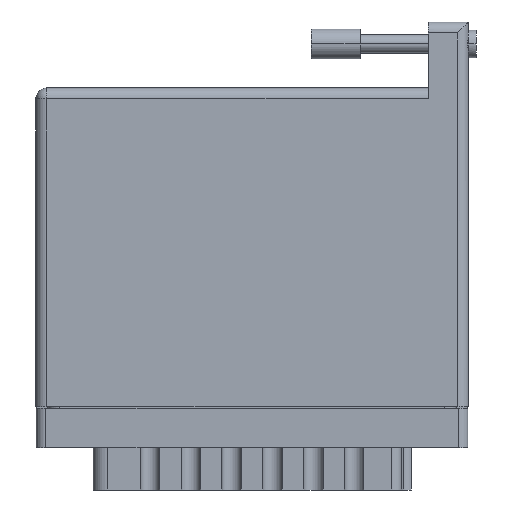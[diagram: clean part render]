
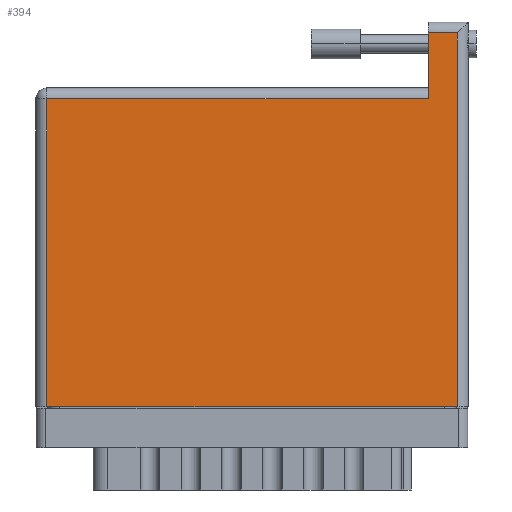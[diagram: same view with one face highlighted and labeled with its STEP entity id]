
A CAD part, front view. The second image highlights one B-rep face of the part: STEP entity #394.
In plain terms, the highlighted face is planar.
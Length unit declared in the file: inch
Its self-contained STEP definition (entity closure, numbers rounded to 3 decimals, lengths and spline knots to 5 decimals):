
#394 = ADVANCED_FACE ( 'NONE', ( #84074 ), #23937, .F. ) ;
#2510 = ORIENTED_EDGE ( 'NONE', *, *, #63102, .T. ) ;
#3109 = ORIENTED_EDGE ( 'NONE', *, *, #71147, .T. ) ;
#5639 = EDGE_CURVE ( 'NONE', #25679, #76016, #22390, .T. ) ;
#7931 = ORIENTED_EDGE ( 'NONE', *, *, #35604, .T. ) ;
#8035 = VERTEX_POINT ( 'NONE', #29273 ) ;
#9094 = DIRECTION ( 'NONE',  ( 0., 1., 0. ) ) ;
#9191 = CARTESIAN_POINT ( 'NONE',  ( 2.685, 0., 0. ) ) ;
#9590 = EDGE_LOOP ( 'NONE', ( #76593, #53223, #57802, #2510, #7931, #3109 ) ) ;
#13926 = VECTOR ( 'NONE', #55453, 39.37008 ) ;
#13989 = CARTESIAN_POINT ( 'NONE',  ( 0.07, 0., 0. ) ) ;
#15470 = CARTESIAN_POINT ( 'NONE',  ( 2.499, 2.45, 0. ) ) ;
#17234 = DIRECTION ( 'NONE',  ( 0., 0., -1. ) ) ;
#18034 = VECTOR ( 'NONE', #61843, 39.37008 ) ;
#18691 = CARTESIAN_POINT ( 'NONE',  ( 2.685, 2.38, 0. ) ) ;
#22390 = LINE ( 'NONE', #89461, #18034 ) ;
#22445 = DIRECTION ( 'NONE',  ( 0., -1., 0. ) ) ;
#23937 = PLANE ( 'NONE',  #67871 ) ;
#25679 = VERTEX_POINT ( 'NONE', #75186 ) ;
#26115 = VECTOR ( 'NONE', #22445, 39.37008 ) ;
#26308 = CARTESIAN_POINT ( 'NONE',  ( 0.07, 0., 0. ) ) ;
#29216 = DIRECTION ( 'NONE',  ( -1., 0., 0. ) ) ;
#29273 = CARTESIAN_POINT ( 'NONE',  ( 2.499, 2.38, 0. ) ) ;
#29654 = CARTESIAN_POINT ( 'NONE',  ( 2.685, 2.45, 0. ) ) ;
#30862 = CARTESIAN_POINT ( 'NONE',  ( 0., 2.03, 0. ) ) ;
#32857 = DIRECTION ( 'NONE',  ( 1., 0., 0. ) ) ;
#35604 = EDGE_CURVE ( 'NONE', #41257, #80407, #88896, .T. ) ;
#36494 = EDGE_CURVE ( 'NONE', #76016, #79771, #86536, .T. ) ;
#41257 = VERTEX_POINT ( 'NONE', #9191 ) ;
#41989 = LINE ( 'NONE', #69802, #72366 ) ;
#44779 = DIRECTION ( 'NONE',  ( -1., 0., 0. ) ) ;
#53223 = ORIENTED_EDGE ( 'NONE', *, *, #5639, .T. ) ;
#55453 = DIRECTION ( 'NONE',  ( 0., -1., 0. ) ) ;
#57802 = ORIENTED_EDGE ( 'NONE', *, *, #36494, .T. ) ;
#59563 = VECTOR ( 'NONE', #9094, 39.37008 ) ;
#60505 = CARTESIAN_POINT ( 'NONE',  ( 0.07, 1.96, 0. ) ) ;
#61034 = CARTESIAN_POINT ( 'NONE',  ( 0., 0., 0. ) ) ;
#61843 = DIRECTION ( 'NONE',  ( -1., 0., 0. ) ) ;
#63102 = EDGE_CURVE ( 'NONE', #79771, #41257, #83924, .T. ) ;
#65100 = LINE ( 'NONE', #15470, #26115 ) ;
#67871 = AXIS2_PLACEMENT_3D ( 'NONE', #30862, #17234, #44779 ) ;
#69802 = CARTESIAN_POINT ( 'NONE',  ( 0., 2.38, 0. ) ) ;
#71147 = EDGE_CURVE ( 'NONE', #80407, #8035, #41989, .T. ) ;
#71994 = VECTOR ( 'NONE', #32857, 39.37008 ) ;
#72366 = VECTOR ( 'NONE', #29216, 39.37008 ) ;
#75186 = CARTESIAN_POINT ( 'NONE',  ( 2.499, 1.96, 0. ) ) ;
#76016 = VERTEX_POINT ( 'NONE', #60505 ) ;
#76593 = ORIENTED_EDGE ( 'NONE', *, *, #77573, .T. ) ;
#77573 = EDGE_CURVE ( 'NONE', #8035, #25679, #65100, .T. ) ;
#79771 = VERTEX_POINT ( 'NONE', #26308 ) ;
#80407 = VERTEX_POINT ( 'NONE', #18691 ) ;
#83924 = LINE ( 'NONE', #61034, #71994 ) ;
#84074 = FACE_OUTER_BOUND ( 'NONE', #9590, .T. ) ;
#86536 = LINE ( 'NONE', #13989, #13926 ) ;
#88896 = LINE ( 'NONE', #29654, #59563 ) ;
#89461 = CARTESIAN_POINT ( 'NONE',  ( 0., 1.96, 0. ) ) ;
